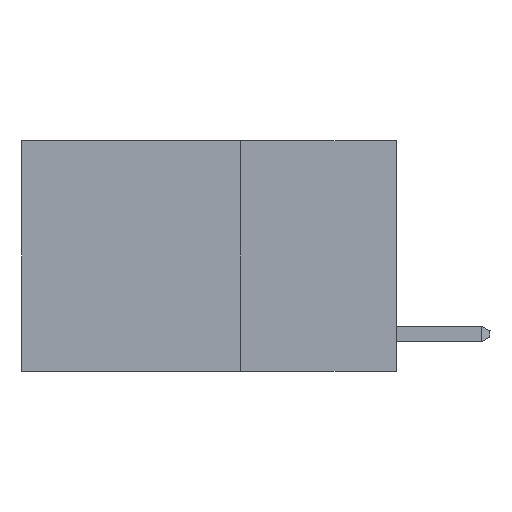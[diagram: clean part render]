
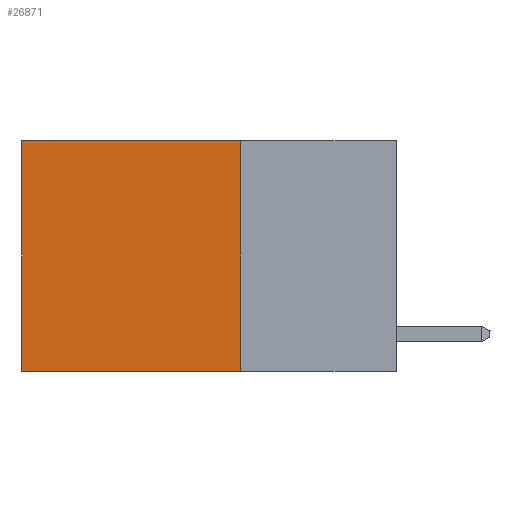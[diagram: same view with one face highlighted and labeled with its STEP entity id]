
A CAD part, left-side view. The second image highlights one B-rep face of the part: STEP entity #26871.
In plain terms, the highlighted planar face has unit normal (-1, 0, 0).
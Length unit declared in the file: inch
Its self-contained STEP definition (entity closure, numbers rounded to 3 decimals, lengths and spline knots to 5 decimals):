
#538 = ORIENTED_EDGE ( 'NONE', *, *, #26632, .F. ) ;
#1380 = CARTESIAN_POINT ( 'NONE',  ( 0.2625, 0.25, 0. ) ) ;
#1471 = VECTOR ( 'NONE', #29285, 39.37008 ) ;
#1800 = DIRECTION ( 'NONE',  ( 0., 1., 0. ) ) ;
#2212 = LINE ( 'NONE', #15824, #1471 ) ;
#3098 = PLANE ( 'NONE',  #6837 ) ;
#3437 = VECTOR ( 'NONE', #22785, 39.37008 ) ;
#6552 = ORIENTED_EDGE ( 'NONE', *, *, #17328, .F. ) ;
#6612 = VECTOR ( 'NONE', #25424, 39.37008 ) ;
#6837 = AXIS2_PLACEMENT_3D ( 'NONE', #1380, #24284, #10214 ) ;
#7889 = EDGE_LOOP ( 'NONE', ( #20071, #6552, #538, #14082 ) ) ;
#10214 = DIRECTION ( 'NONE',  ( 0., 0., -1. ) ) ;
#13233 = LINE ( 'NONE', #17765, #3437 ) ;
#13679 = CARTESIAN_POINT ( 'NONE',  ( 0.2625, 0.6, 0. ) ) ;
#14072 = CARTESIAN_POINT ( 'NONE',  ( 0.2625, 0.25, 0. ) ) ;
#14082 = ORIENTED_EDGE ( 'NONE', *, *, #19596, .T. ) ;
#14517 = LINE ( 'NONE', #14072, #6612 ) ;
#15121 = CARTESIAN_POINT ( 'NONE',  ( 0.2625, 0.6, -0.37 ) ) ;
#15220 = VECTOR ( 'NONE', #1800, 39.37008 ) ;
#15824 = CARTESIAN_POINT ( 'NONE',  ( 0.2625, 0.25, 0. ) ) ;
#17328 = EDGE_CURVE ( 'NONE', #18932, #24750, #22720, .T. ) ;
#17765 = CARTESIAN_POINT ( 'NONE',  ( 0.2625, 0.6, 0. ) ) ;
#18932 = VERTEX_POINT ( 'NONE', #26897 ) ;
#19596 = EDGE_CURVE ( 'NONE', #25236, #28694, #14517, .T. ) ;
#19753 = FACE_OUTER_BOUND ( 'NONE', #7889, .T. ) ;
#20071 = ORIENTED_EDGE ( 'NONE', *, *, #26953, .T. ) ;
#22720 = LINE ( 'NONE', #26926, #15220 ) ;
#22785 = DIRECTION ( 'NONE',  ( 0., 0., -1. ) ) ;
#24284 = DIRECTION ( 'NONE',  ( 1., 0., 0. ) ) ;
#24750 = VERTEX_POINT ( 'NONE', #15121 ) ;
#24761 = CARTESIAN_POINT ( 'NONE',  ( 0.2625, 0.25, 0. ) ) ;
#25236 = VERTEX_POINT ( 'NONE', #24761 ) ;
#25424 = DIRECTION ( 'NONE',  ( 0., 1., 0. ) ) ;
#26632 = EDGE_CURVE ( 'NONE', #25236, #18932, #2212, .T. ) ;
#26871 = ADVANCED_FACE ( 'NONE', ( #19753 ), #3098, .F. ) ;
#26897 = CARTESIAN_POINT ( 'NONE',  ( 0.2625, 0.25, -0.37 ) ) ;
#26926 = CARTESIAN_POINT ( 'NONE',  ( 0.2625, 0.25, -0.37 ) ) ;
#26953 = EDGE_CURVE ( 'NONE', #28694, #24750, #13233, .T. ) ;
#28694 = VERTEX_POINT ( 'NONE', #13679 ) ;
#29285 = DIRECTION ( 'NONE',  ( 0., 0., -1. ) ) ;
